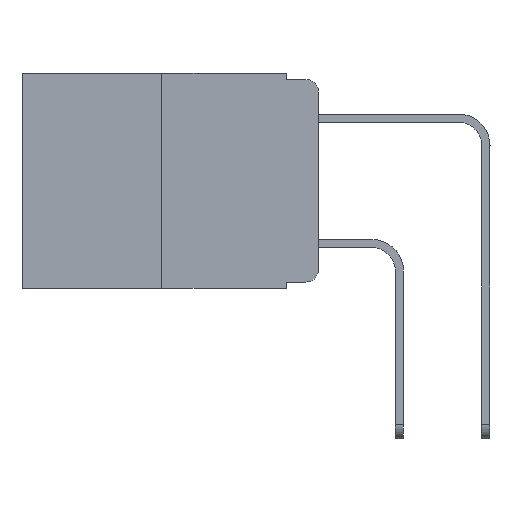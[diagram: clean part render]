
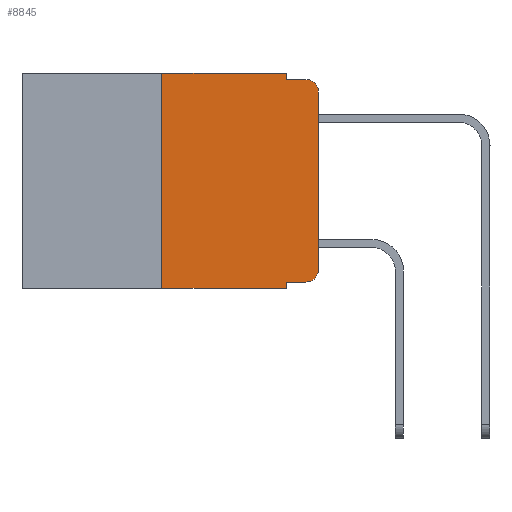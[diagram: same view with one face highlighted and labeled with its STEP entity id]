
A CAD part, left-side view. The second image highlights one B-rep face of the part: STEP entity #8845.
In plain terms, the highlighted planar face has unit normal (-1, 0, 0).
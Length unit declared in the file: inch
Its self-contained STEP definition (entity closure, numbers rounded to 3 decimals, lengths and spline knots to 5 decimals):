
#96 = CARTESIAN_POINT ( 'NONE',  ( 0., 0.02, -0.01 ) ) ;
#174 = VERTEX_POINT ( 'NONE', #7736 ) ;
#176 = ORIENTED_EDGE ( 'NONE', *, *, #6384, .F. ) ;
#280 = VECTOR ( 'NONE', #1326, 39.37008 ) ;
#565 = CARTESIAN_POINT ( 'NONE',  ( 0., 0.473, 0. ) ) ;
#656 = VERTEX_POINT ( 'NONE', #7499 ) ;
#763 = LINE ( 'NONE', #565, #6808 ) ;
#775 = EDGE_CURVE ( 'NONE', #2918, #5009, #11807, .T. ) ;
#808 = EDGE_CURVE ( 'NONE', #9941, #2918, #10142, .T. ) ;
#1056 = VERTEX_POINT ( 'NONE', #9685 ) ;
#1067 = EDGE_CURVE ( 'NONE', #4784, #5009, #5023, .T. ) ;
#1168 = VECTOR ( 'NONE', #7096, 39.37008 ) ;
#1326 = DIRECTION ( 'NONE',  ( 0., 0., 1. ) ) ;
#1457 = CARTESIAN_POINT ( 'NONE',  ( 0., 0.25, 0. ) ) ;
#1706 = CARTESIAN_POINT ( 'NONE',  ( 0., 0.25, -0.343 ) ) ;
#1750 = DIRECTION ( 'NONE',  ( 0., -1., 0. ) ) ;
#1781 = DIRECTION ( 'NONE',  ( 0., -1., 0. ) ) ;
#1864 = DIRECTION ( 'NONE',  ( -1., 0., 0. ) ) ;
#2025 = VERTEX_POINT ( 'NONE', #10743 ) ;
#2547 = FACE_OUTER_BOUND ( 'NONE', #8637, .T. ) ;
#2563 = LINE ( 'NONE', #2829, #7985 ) ;
#2829 = CARTESIAN_POINT ( 'NONE',  ( 0., 0.051, 0. ) ) ;
#2832 = CARTESIAN_POINT ( 'NONE',  ( 0., 0.051, -0.343 ) ) ;
#2918 = VERTEX_POINT ( 'NONE', #8942 ) ;
#2953 = LINE ( 'NONE', #7185, #1168 ) ;
#3043 = CARTESIAN_POINT ( 'NONE',  ( 0., 0., 0. ) ) ;
#3191 = ORIENTED_EDGE ( 'NONE', *, *, #9095, .F. ) ;
#3483 = CARTESIAN_POINT ( 'NONE',  ( 0., 0.473, -0.343 ) ) ;
#3778 = EDGE_CURVE ( 'NONE', #174, #2025, #5781, .T. ) ;
#3796 = LINE ( 'NONE', #3483, #7418 ) ;
#4164 = EDGE_CURVE ( 'NONE', #2025, #9941, #6772, .T. ) ;
#4443 = ORIENTED_EDGE ( 'NONE', *, *, #1067, .F. ) ;
#4784 = VERTEX_POINT ( 'NONE', #6107 ) ;
#5009 = VERTEX_POINT ( 'NONE', #96 ) ;
#5023 = LINE ( 'NONE', #13420, #5675 ) ;
#5129 = DIRECTION ( 'NONE',  ( 0., 0., -1. ) ) ;
#5222 = DIRECTION ( 'NONE',  ( 0., 0., -1. ) ) ;
#5572 = AXIS2_PLACEMENT_3D ( 'NONE', #8833, #9819, #7656 ) ;
#5675 = VECTOR ( 'NONE', #1781, 39.37008 ) ;
#5781 = LINE ( 'NONE', #9107, #7766 ) ;
#6056 = DIRECTION ( 'NONE',  ( 0., -1., 0. ) ) ;
#6107 = CARTESIAN_POINT ( 'NONE',  ( 0., 0.051, -0.01 ) ) ;
#6206 = ORIENTED_EDGE ( 'NONE', *, *, #3778, .T. ) ;
#6384 = EDGE_CURVE ( 'NONE', #1056, #4784, #2953, .T. ) ;
#6563 = PLANE ( 'NONE',  #5572 ) ;
#6772 = CIRCLE ( 'NONE', #6950, 0.02 ) ;
#6808 = VECTOR ( 'NONE', #1750, 39.37008 ) ;
#6950 = AXIS2_PLACEMENT_3D ( 'NONE', #10456, #10326, #5222 ) ;
#7096 = DIRECTION ( 'NONE',  ( 0., 0., -1. ) ) ;
#7185 = CARTESIAN_POINT ( 'NONE',  ( 0., 0.051, 0. ) ) ;
#7232 = ORIENTED_EDGE ( 'NONE', *, *, #8721, .F. ) ;
#7261 = DIRECTION ( 'NONE',  ( 0., 0., 1. ) ) ;
#7418 = VECTOR ( 'NONE', #10831, 39.37008 ) ;
#7499 = CARTESIAN_POINT ( 'NONE',  ( 0., 0.25, 0. ) ) ;
#7656 = DIRECTION ( 'NONE',  ( 0., 0., -1. ) ) ;
#7658 = LINE ( 'NONE', #1457, #280 ) ;
#7736 = CARTESIAN_POINT ( 'NONE',  ( 0., 0.051, -0.333 ) ) ;
#7766 = VECTOR ( 'NONE', #6056, 39.37008 ) ;
#7878 = ORIENTED_EDGE ( 'NONE', *, *, #4164, .T. ) ;
#7985 = VECTOR ( 'NONE', #10159, 39.37008 ) ;
#8172 = AXIS2_PLACEMENT_3D ( 'NONE', #9304, #1864, #5129 ) ;
#8174 = ORIENTED_EDGE ( 'NONE', *, *, #10355, .T. ) ;
#8514 = VECTOR ( 'NONE', #7261, 39.37008 ) ;
#8637 = EDGE_LOOP ( 'NONE', ( #11916, #8841, #4443, #176, #3191, #13231, #8174, #7232, #6206, #7878 ) ) ;
#8721 = EDGE_CURVE ( 'NONE', #174, #11732, #2563, .T. ) ;
#8833 = CARTESIAN_POINT ( 'NONE',  ( 0., 0.473, 0. ) ) ;
#8841 = ORIENTED_EDGE ( 'NONE', *, *, #775, .T. ) ;
#8845 = ADVANCED_FACE ( 'NONE', ( #2547 ), #6563, .F. ) ;
#8942 = CARTESIAN_POINT ( 'NONE',  ( 0., 0., -0.03 ) ) ;
#9095 = EDGE_CURVE ( 'NONE', #656, #1056, #763, .T. ) ;
#9107 = CARTESIAN_POINT ( 'NONE',  ( 0., 0.051, -0.333 ) ) ;
#9226 = VERTEX_POINT ( 'NONE', #1706 ) ;
#9304 = CARTESIAN_POINT ( 'NONE',  ( 0., 0.02, -0.03 ) ) ;
#9685 = CARTESIAN_POINT ( 'NONE',  ( 0., 0.051, 0. ) ) ;
#9819 = DIRECTION ( 'NONE',  ( 1., 0., 0. ) ) ;
#9941 = VERTEX_POINT ( 'NONE', #10072 ) ;
#10072 = CARTESIAN_POINT ( 'NONE',  ( 0., 0., -0.313 ) ) ;
#10142 = LINE ( 'NONE', #3043, #8514 ) ;
#10159 = DIRECTION ( 'NONE',  ( 0., 0., -1. ) ) ;
#10326 = DIRECTION ( 'NONE',  ( -1., 0., 0. ) ) ;
#10355 = EDGE_CURVE ( 'NONE', #9226, #11732, #3796, .T. ) ;
#10456 = CARTESIAN_POINT ( 'NONE',  ( 0., 0.02, -0.313 ) ) ;
#10743 = CARTESIAN_POINT ( 'NONE',  ( 0., 0.02, -0.333 ) ) ;
#10831 = DIRECTION ( 'NONE',  ( 0., -1., 0. ) ) ;
#11732 = VERTEX_POINT ( 'NONE', #2832 ) ;
#11807 = CIRCLE ( 'NONE', #8172, 0.02 ) ;
#11916 = ORIENTED_EDGE ( 'NONE', *, *, #808, .T. ) ;
#13190 = EDGE_CURVE ( 'NONE', #9226, #656, #7658, .T. ) ;
#13231 = ORIENTED_EDGE ( 'NONE', *, *, #13190, .F. ) ;
#13420 = CARTESIAN_POINT ( 'NONE',  ( 0., 0.051, -0.01 ) ) ;
